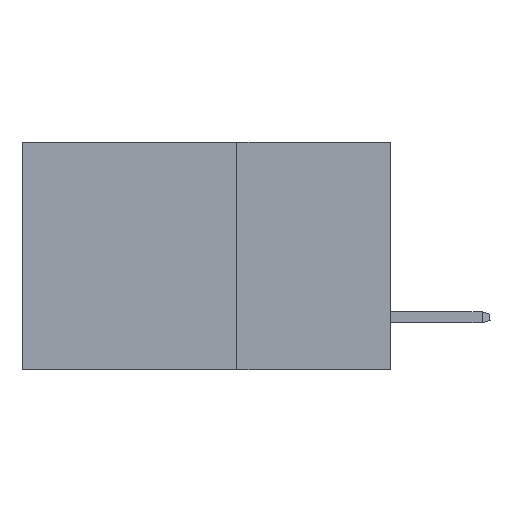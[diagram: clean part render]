
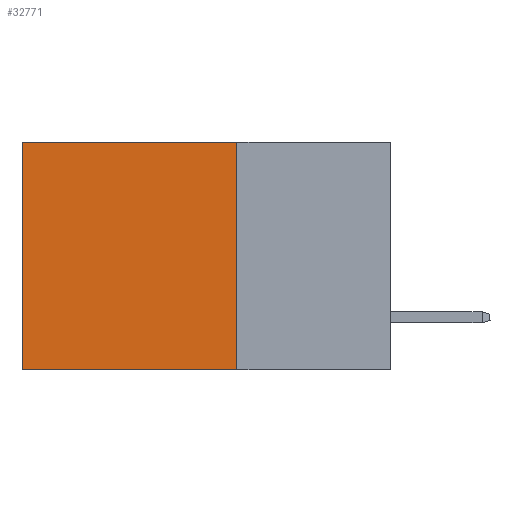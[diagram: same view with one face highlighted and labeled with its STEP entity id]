
A CAD part, left-side view. The second image highlights one B-rep face of the part: STEP entity #32771.
In plain terms, the highlighted planar face has unit normal (-1, 0, 0).
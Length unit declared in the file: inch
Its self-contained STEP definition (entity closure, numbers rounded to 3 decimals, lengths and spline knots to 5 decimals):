
#1102 = VECTOR ( 'NONE', #36222, 39.37008 ) ;
#1242 = CARTESIAN_POINT ( 'NONE',  ( 0.2875, 0.6, 0. ) ) ;
#2814 = DIRECTION ( 'NONE',  ( 0., 0., -1. ) ) ;
#3799 = VERTEX_POINT ( 'NONE', #24511 ) ;
#5276 = CARTESIAN_POINT ( 'NONE',  ( 0.2875, 0.25, 0. ) ) ;
#5657 = VECTOR ( 'NONE', #9497, 39.37008 ) ;
#5986 = AXIS2_PLACEMENT_3D ( 'NONE', #12789, #28492, #2814 ) ;
#7071 = EDGE_CURVE ( 'NONE', #40167, #34918, #39179, .T. ) ;
#7699 = LINE ( 'NONE', #28878, #5657 ) ;
#9497 = DIRECTION ( 'NONE',  ( 0., 1., 0. ) ) ;
#9792 = LINE ( 'NONE', #1242, #1102 ) ;
#10144 = CARTESIAN_POINT ( 'NONE',  ( 0.2875, 0.25, 0. ) ) ;
#10743 = VECTOR ( 'NONE', #34222, 39.37008 ) ;
#12789 = CARTESIAN_POINT ( 'NONE',  ( 0.2875, 0.25, 0. ) ) ;
#16174 = EDGE_CURVE ( 'NONE', #40167, #3799, #38934, .T. ) ;
#17204 = DIRECTION ( 'NONE',  ( 0., 0., -1. ) ) ;
#20181 = FACE_OUTER_BOUND ( 'NONE', #23026, .T. ) ;
#22538 = PLANE ( 'NONE',  #5986 ) ;
#22947 = CARTESIAN_POINT ( 'NONE',  ( 0.2875, 0.6, -0.37 ) ) ;
#23026 = EDGE_LOOP ( 'NONE', ( #28845, #30926, #41513, #39993 ) ) ;
#24511 = CARTESIAN_POINT ( 'NONE',  ( 0.2875, 0.25, -0.37 ) ) ;
#28492 = DIRECTION ( 'NONE',  ( 1., 0., 0. ) ) ;
#28745 = EDGE_CURVE ( 'NONE', #3799, #38283, #7699, .T. ) ;
#28845 = ORIENTED_EDGE ( 'NONE', *, *, #42059, .T. ) ;
#28878 = CARTESIAN_POINT ( 'NONE',  ( 0.2875, 0.25, -0.37 ) ) ;
#30075 = CARTESIAN_POINT ( 'NONE',  ( 0.2875, 0.25, 0. ) ) ;
#30926 = ORIENTED_EDGE ( 'NONE', *, *, #28745, .F. ) ;
#32771 = ADVANCED_FACE ( 'NONE', ( #20181 ), #22538, .F. ) ;
#34222 = DIRECTION ( 'NONE',  ( 0., 1., 0. ) ) ;
#34918 = VERTEX_POINT ( 'NONE', #38651 ) ;
#36222 = DIRECTION ( 'NONE',  ( 0., 0., -1. ) ) ;
#38283 = VERTEX_POINT ( 'NONE', #22947 ) ;
#38651 = CARTESIAN_POINT ( 'NONE',  ( 0.2875, 0.6, 0. ) ) ;
#38934 = LINE ( 'NONE', #30075, #40988 ) ;
#39179 = LINE ( 'NONE', #5276, #10743 ) ;
#39993 = ORIENTED_EDGE ( 'NONE', *, *, #7071, .T. ) ;
#40167 = VERTEX_POINT ( 'NONE', #10144 ) ;
#40988 = VECTOR ( 'NONE', #17204, 39.37008 ) ;
#41513 = ORIENTED_EDGE ( 'NONE', *, *, #16174, .F. ) ;
#42059 = EDGE_CURVE ( 'NONE', #34918, #38283, #9792, .T. ) ;
